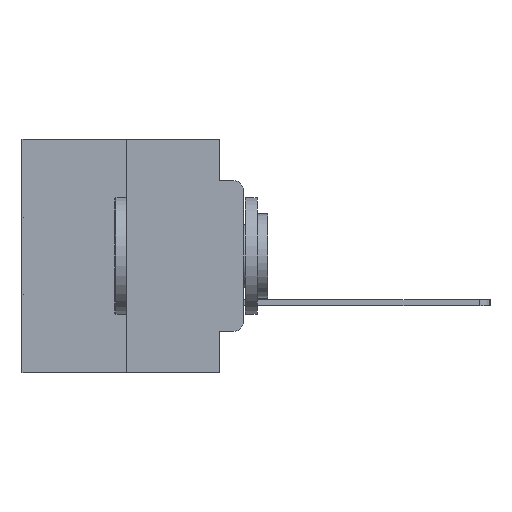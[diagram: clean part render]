
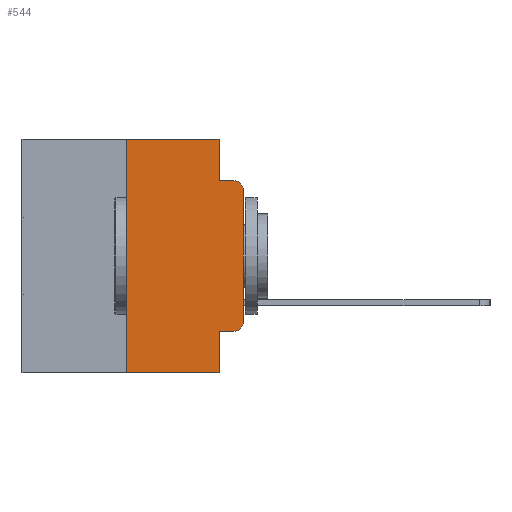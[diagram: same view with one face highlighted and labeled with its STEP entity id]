
A CAD part, left-side view. The second image highlights one B-rep face of the part: STEP entity #544.
In plain terms, the highlighted planar face has unit normal (-1, 0, 0).
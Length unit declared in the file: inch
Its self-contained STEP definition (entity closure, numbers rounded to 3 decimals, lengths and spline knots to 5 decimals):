
#102 = VERTEX_POINT ( 'NONE', #27743 ) ;
#426 = DIRECTION ( 'NONE',  ( 0., -1., 0. ) ) ;
#544 = ADVANCED_FACE ( 'NONE', ( #12059 ), #22782, .F. ) ;
#1296 = CARTESIAN_POINT ( 'NONE',  ( 0., 0.051, 0. ) ) ;
#1441 = EDGE_CURVE ( 'NONE', #7649, #3574, #6576, .T. ) ;
#1641 = VECTOR ( 'NONE', #5747, 39.37008 ) ;
#2336 = LINE ( 'NONE', #26123, #1641 ) ;
#2542 = CARTESIAN_POINT ( 'NONE',  ( 0., 0.051, -0.4115 ) ) ;
#2549 = CARTESIAN_POINT ( 'NONE',  ( 0., 0.02, -0.1085 ) ) ;
#2558 = CARTESIAN_POINT ( 'NONE',  ( 0., 0.25, 0. ) ) ;
#2792 = CARTESIAN_POINT ( 'NONE',  ( 0., 0., -0.3915 ) ) ;
#3079 = LINE ( 'NONE', #2542, #25910 ) ;
#3202 = VERTEX_POINT ( 'NONE', #2558 ) ;
#3574 = VERTEX_POINT ( 'NONE', #13096 ) ;
#3680 = CARTESIAN_POINT ( 'NONE',  ( 0., 0.02, -0.4115 ) ) ;
#4394 = VERTEX_POINT ( 'NONE', #2792 ) ;
#4440 = EDGE_CURVE ( 'NONE', #26356, #102, #17372, .T. ) ;
#4534 = EDGE_CURVE ( 'NONE', #4394, #7649, #2336, .T. ) ;
#4897 = DIRECTION ( 'NONE',  ( 0., 0., -1. ) ) ;
#5481 = VECTOR ( 'NONE', #14810, 39.37008 ) ;
#5747 = DIRECTION ( 'NONE',  ( 0., 0., 1. ) ) ;
#6068 = EDGE_LOOP ( 'NONE', ( #23893, #23783, #18551, #19103, #24420, #24478, #24531, #26445, #26502, #25854 ) ) ;
#6443 = LINE ( 'NONE', #1296, #11864 ) ;
#6576 = CIRCLE ( 'NONE', #29047, 0.02 ) ;
#7087 = CARTESIAN_POINT ( 'NONE',  ( 0., 0.051, 0. ) ) ;
#7423 = AXIS2_PLACEMENT_3D ( 'NONE', #23738, #10288, #26028 ) ;
#7649 = VERTEX_POINT ( 'NONE', #20893 ) ;
#8242 = CIRCLE ( 'NONE', #7423, 0.02 ) ;
#9110 = VERTEX_POINT ( 'NONE', #3680 ) ;
#10022 = LINE ( 'NONE', #28989, #21252 ) ;
#10288 = DIRECTION ( 'NONE',  ( -1., 0., 0. ) ) ;
#10358 = LINE ( 'NONE', #12012, #20871 ) ;
#11405 = VECTOR ( 'NONE', #27493, 39.37008 ) ;
#11864 = VECTOR ( 'NONE', #21883, 39.37008 ) ;
#12012 = CARTESIAN_POINT ( 'NONE',  ( 0., 0.473, 0. ) ) ;
#12059 = FACE_OUTER_BOUND ( 'NONE', #6068, .T. ) ;
#13096 = CARTESIAN_POINT ( 'NONE',  ( 0., 0.02, -0.0885 ) ) ;
#14810 = DIRECTION ( 'NONE',  ( 0., 0., 1. ) ) ;
#15024 = VERTEX_POINT ( 'NONE', #7087 ) ;
#15832 = EDGE_CURVE ( 'NONE', #9110, #4394, #8242, .T. ) ;
#16125 = VERTEX_POINT ( 'NONE', #29252 ) ;
#16402 = DIRECTION ( 'NONE',  ( 0., 0., -1. ) ) ;
#16675 = VECTOR ( 'NONE', #18970, 39.37008 ) ;
#16702 = CARTESIAN_POINT ( 'NONE',  ( 0., 0.473, -0.5 ) ) ;
#17372 = LINE ( 'NONE', #16702, #16675 ) ;
#18536 = DIRECTION ( 'NONE',  ( -1., 0., 0. ) ) ;
#18551 = ORIENTED_EDGE ( 'NONE', *, *, #29365, .F. ) ;
#18970 = DIRECTION ( 'NONE',  ( 0., -1., 0. ) ) ;
#19103 = ORIENTED_EDGE ( 'NONE', *, *, #27924, .F. ) ;
#20061 = DIRECTION ( 'NONE',  ( 0., 0., -1. ) ) ;
#20215 = VERTEX_POINT ( 'NONE', #25969 ) ;
#20834 = DIRECTION ( 'NONE',  ( 0., -1., 0. ) ) ;
#20871 = VECTOR ( 'NONE', #426, 39.37008 ) ;
#20893 = CARTESIAN_POINT ( 'NONE',  ( 0., 0., -0.1085 ) ) ;
#21252 = VECTOR ( 'NONE', #20061, 39.37008 ) ;
#21883 = DIRECTION ( 'NONE',  ( 0., 0., -1. ) ) ;
#21918 = EDGE_CURVE ( 'NONE', #16125, #9110, #3079, .T. ) ;
#22743 = DIRECTION ( 'NONE',  ( 1., 0., 0. ) ) ;
#22782 = PLANE ( 'NONE',  #27751 ) ;
#23366 = LINE ( 'NONE', #25245, #11405 ) ;
#23397 = EDGE_CURVE ( 'NONE', #16125, #102, #10022, .T. ) ;
#23665 = EDGE_CURVE ( 'NONE', #3202, #15024, #10358, .T. ) ;
#23738 = CARTESIAN_POINT ( 'NONE',  ( 0., 0.02, -0.3915 ) ) ;
#23783 = ORIENTED_EDGE ( 'NONE', *, *, #1441, .T. ) ;
#23893 = ORIENTED_EDGE ( 'NONE', *, *, #4534, .T. ) ;
#24333 = LINE ( 'NONE', #26090, #5481 ) ;
#24420 = ORIENTED_EDGE ( 'NONE', *, *, #23665, .F. ) ;
#24478 = ORIENTED_EDGE ( 'NONE', *, *, #24924, .F. ) ;
#24531 = ORIENTED_EDGE ( 'NONE', *, *, #4440, .T. ) ;
#24924 = EDGE_CURVE ( 'NONE', #26356, #3202, #24333, .T. ) ;
#25021 = CARTESIAN_POINT ( 'NONE',  ( 0., 0.473, 0. ) ) ;
#25245 = CARTESIAN_POINT ( 'NONE',  ( 0., 0.051, -0.0885 ) ) ;
#25854 = ORIENTED_EDGE ( 'NONE', *, *, #15832, .T. ) ;
#25910 = VECTOR ( 'NONE', #20834, 39.37008 ) ;
#25969 = CARTESIAN_POINT ( 'NONE',  ( 0., 0.051, -0.0885 ) ) ;
#26028 = DIRECTION ( 'NONE',  ( 0., 0., -1. ) ) ;
#26090 = CARTESIAN_POINT ( 'NONE',  ( 0., 0.25, 0. ) ) ;
#26123 = CARTESIAN_POINT ( 'NONE',  ( 0., 0., 0. ) ) ;
#26356 = VERTEX_POINT ( 'NONE', #27083 ) ;
#26445 = ORIENTED_EDGE ( 'NONE', *, *, #23397, .F. ) ;
#26502 = ORIENTED_EDGE ( 'NONE', *, *, #21918, .T. ) ;
#27083 = CARTESIAN_POINT ( 'NONE',  ( 0., 0.25, -0.5 ) ) ;
#27493 = DIRECTION ( 'NONE',  ( 0., -1., 0. ) ) ;
#27743 = CARTESIAN_POINT ( 'NONE',  ( 0., 0.051, -0.5 ) ) ;
#27751 = AXIS2_PLACEMENT_3D ( 'NONE', #25021, #22743, #16402 ) ;
#27924 = EDGE_CURVE ( 'NONE', #15024, #20215, #6443, .T. ) ;
#28989 = CARTESIAN_POINT ( 'NONE',  ( 0., 0.051, 0. ) ) ;
#29047 = AXIS2_PLACEMENT_3D ( 'NONE', #2549, #18536, #4897 ) ;
#29252 = CARTESIAN_POINT ( 'NONE',  ( 0., 0.051, -0.4115 ) ) ;
#29365 = EDGE_CURVE ( 'NONE', #20215, #3574, #23366, .T. ) ;
